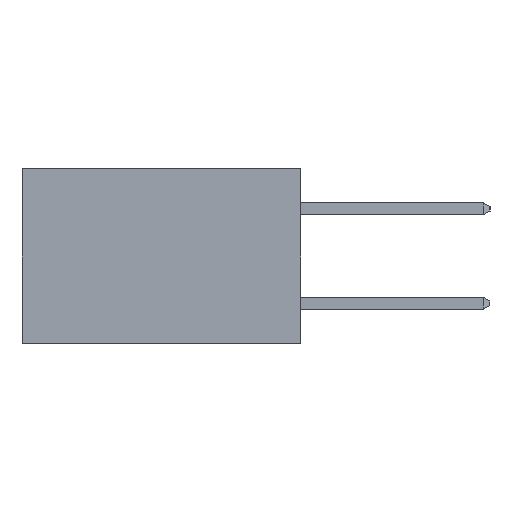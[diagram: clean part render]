
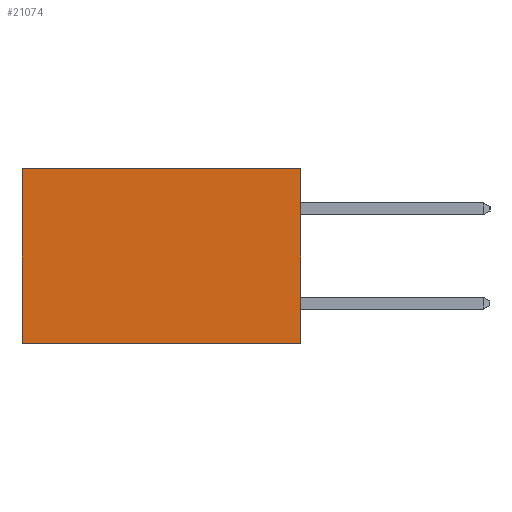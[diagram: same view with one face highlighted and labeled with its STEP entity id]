
A CAD part, left-side view. The second image highlights one B-rep face of the part: STEP entity #21074.
In plain terms, the highlighted planar face has unit normal (-1, 0, 0).
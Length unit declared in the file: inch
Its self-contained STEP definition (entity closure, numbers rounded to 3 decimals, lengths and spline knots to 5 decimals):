
#489 = EDGE_CURVE ( 'NONE', #17673, #21481, #29810, .T. ) ;
#2096 = DIRECTION ( 'NONE',  ( 0., 1., 0. ) ) ;
#2368 = CARTESIAN_POINT ( 'NONE',  ( 0.277, 0., -0.37 ) ) ;
#3253 = VECTOR ( 'NONE', #2096, 39.37008 ) ;
#4153 = ORIENTED_EDGE ( 'NONE', *, *, #10700, .T. ) ;
#4704 = EDGE_CURVE ( 'NONE', #21481, #6510, #29254, .T. ) ;
#4733 = DIRECTION ( 'NONE',  ( 1., 0., 0. ) ) ;
#6510 = VERTEX_POINT ( 'NONE', #7334 ) ;
#7030 = EDGE_CURVE ( 'NONE', #14931, #6510, #24408, .T. ) ;
#7187 = VECTOR ( 'NONE', #26213, 39.37008 ) ;
#7334 = CARTESIAN_POINT ( 'NONE',  ( 0.277, 0.59, -0.37 ) ) ;
#7600 = ORIENTED_EDGE ( 'NONE', *, *, #4704, .F. ) ;
#9452 = ORIENTED_EDGE ( 'NONE', *, *, #489, .F. ) ;
#9553 = LINE ( 'NONE', #18553, #3253 ) ;
#10011 = VECTOR ( 'NONE', #12079, 39.37008 ) ;
#10700 = EDGE_CURVE ( 'NONE', #17673, #14931, #9553, .T. ) ;
#11344 = VECTOR ( 'NONE', #13273, 39.37008 ) ;
#12079 = DIRECTION ( 'NONE',  ( 0., 1., 0. ) ) ;
#12413 = CARTESIAN_POINT ( 'NONE',  ( 0.277, 0., -0.37 ) ) ;
#13273 = DIRECTION ( 'NONE',  ( 0., 0., -1. ) ) ;
#14931 = VERTEX_POINT ( 'NONE', #22530 ) ;
#15547 = CARTESIAN_POINT ( 'NONE',  ( 0.277, 0., -0.37 ) ) ;
#17673 = VERTEX_POINT ( 'NONE', #18867 ) ;
#18333 = ORIENTED_EDGE ( 'NONE', *, *, #7030, .T. ) ;
#18553 = CARTESIAN_POINT ( 'NONE',  ( 0.277, 0., 0. ) ) ;
#18867 = CARTESIAN_POINT ( 'NONE',  ( 0.277, 0., 0. ) ) ;
#19089 = EDGE_LOOP ( 'NONE', ( #18333, #7600, #9452, #4153 ) ) ;
#21074 = ADVANCED_FACE ( 'NONE', ( #23676 ), #24091, .F. ) ;
#21156 = DIRECTION ( 'NONE',  ( 0., 0., -1. ) ) ;
#21481 = VERTEX_POINT ( 'NONE', #15547 ) ;
#22523 = CARTESIAN_POINT ( 'NONE',  ( 0.277, 0., -0.37 ) ) ;
#22530 = CARTESIAN_POINT ( 'NONE',  ( 0.277, 0.59, 0. ) ) ;
#23676 = FACE_OUTER_BOUND ( 'NONE', #19089, .T. ) ;
#24091 = PLANE ( 'NONE',  #26509 ) ;
#24408 = LINE ( 'NONE', #26185, #7187 ) ;
#26185 = CARTESIAN_POINT ( 'NONE',  ( 0.277, 0.59, -0.37 ) ) ;
#26213 = DIRECTION ( 'NONE',  ( 0., 0., -1. ) ) ;
#26509 = AXIS2_PLACEMENT_3D ( 'NONE', #2368, #4733, #21156 ) ;
#29254 = LINE ( 'NONE', #12413, #10011 ) ;
#29810 = LINE ( 'NONE', #22523, #11344 ) ;
